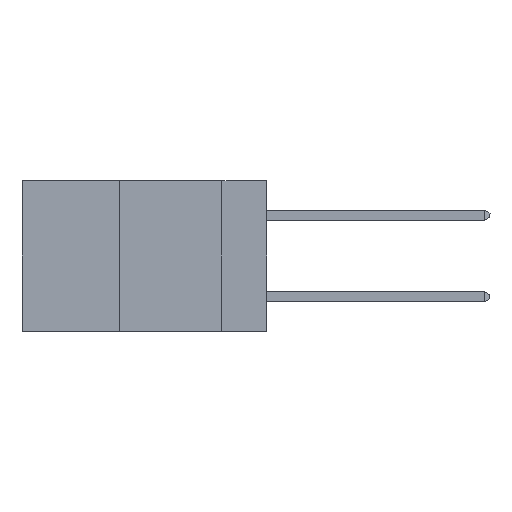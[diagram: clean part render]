
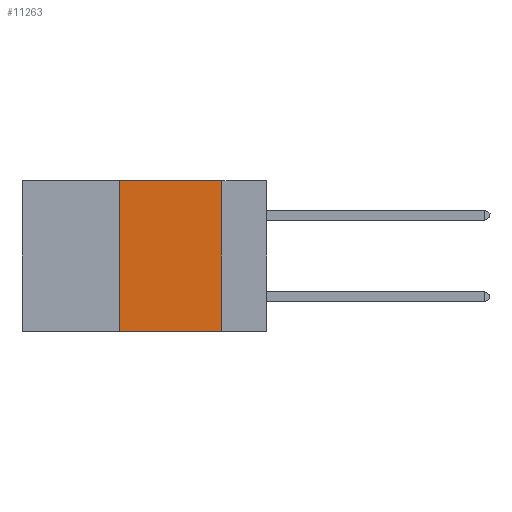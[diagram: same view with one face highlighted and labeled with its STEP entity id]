
A CAD part, left-side view. The second image highlights one B-rep face of the part: STEP entity #11263.
In plain terms, the highlighted planar face has unit normal (-1, 0, 0).
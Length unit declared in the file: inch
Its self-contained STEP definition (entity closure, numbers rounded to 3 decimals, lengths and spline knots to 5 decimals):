
#659 = DIRECTION ( 'NONE',  ( 0., -1., 0. ) ) ;
#1354 = EDGE_CURVE ( 'NONE', #13161, #7188, #9138, .T. ) ;
#1908 = CARTESIAN_POINT ( 'NONE',  ( 0., 0.36, 0. ) ) ;
#2062 = CARTESIAN_POINT ( 'NONE',  ( 0., 0.11, -0.37 ) ) ;
#2161 = DIRECTION ( 'NONE',  ( 0., -1., 0. ) ) ;
#2460 = CARTESIAN_POINT ( 'NONE',  ( 0., 0.6, -0.37 ) ) ;
#2666 = CARTESIAN_POINT ( 'NONE',  ( 0., 0.11, 0. ) ) ;
#2694 = PLANE ( 'NONE',  #9593 ) ;
#3554 = VERTEX_POINT ( 'NONE', #2062 ) ;
#3600 = ORIENTED_EDGE ( 'NONE', *, *, #1354, .F. ) ;
#3829 = DIRECTION ( 'NONE',  ( 1., 0., 0. ) ) ;
#4194 = EDGE_CURVE ( 'NONE', #7188, #3554, #9137, .T. ) ;
#4974 = VECTOR ( 'NONE', #12256, 39.37008 ) ;
#4978 = EDGE_CURVE ( 'NONE', #7628, #3554, #12204, .T. ) ;
#5153 = VECTOR ( 'NONE', #659, 39.37008 ) ;
#6140 = EDGE_LOOP ( 'NONE', ( #14251, #3600, #10209, #7281 ) ) ;
#6321 = CARTESIAN_POINT ( 'NONE',  ( 0., 0.11, 0. ) ) ;
#7188 = VERTEX_POINT ( 'NONE', #2666 ) ;
#7281 = ORIENTED_EDGE ( 'NONE', *, *, #4978, .T. ) ;
#7628 = VERTEX_POINT ( 'NONE', #8802 ) ;
#8802 = CARTESIAN_POINT ( 'NONE',  ( 0., 0.36, -0.37 ) ) ;
#9000 = DIRECTION ( 'NONE',  ( 0., 0., -1. ) ) ;
#9137 = LINE ( 'NONE', #6321, #4974 ) ;
#9138 = LINE ( 'NONE', #14262, #5153 ) ;
#9410 = EDGE_CURVE ( 'NONE', #7628, #13161, #9514, .T. ) ;
#9438 = CARTESIAN_POINT ( 'NONE',  ( 0., 0.36, 0. ) ) ;
#9514 = LINE ( 'NONE', #9438, #9823 ) ;
#9593 = AXIS2_PLACEMENT_3D ( 'NONE', #10227, #3829, #9000 ) ;
#9823 = VECTOR ( 'NONE', #14476, 39.37008 ) ;
#10209 = ORIENTED_EDGE ( 'NONE', *, *, #9410, .F. ) ;
#10227 = CARTESIAN_POINT ( 'NONE',  ( 0., 0.6, 0. ) ) ;
#11263 = ADVANCED_FACE ( 'NONE', ( #15266 ), #2694, .F. ) ;
#12204 = LINE ( 'NONE', #2460, #13552 ) ;
#12256 = DIRECTION ( 'NONE',  ( 0., 0., -1. ) ) ;
#13161 = VERTEX_POINT ( 'NONE', #1908 ) ;
#13552 = VECTOR ( 'NONE', #2161, 39.37008 ) ;
#14251 = ORIENTED_EDGE ( 'NONE', *, *, #4194, .F. ) ;
#14262 = CARTESIAN_POINT ( 'NONE',  ( 0., 0.6, 0. ) ) ;
#14476 = DIRECTION ( 'NONE',  ( 0., 0., 1. ) ) ;
#15266 = FACE_OUTER_BOUND ( 'NONE', #6140, .T. ) ;
